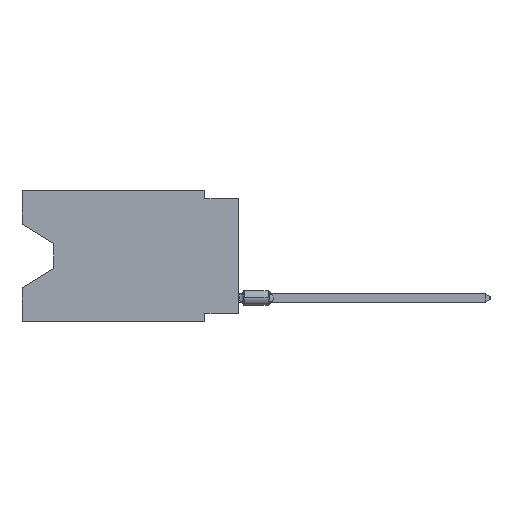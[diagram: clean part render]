
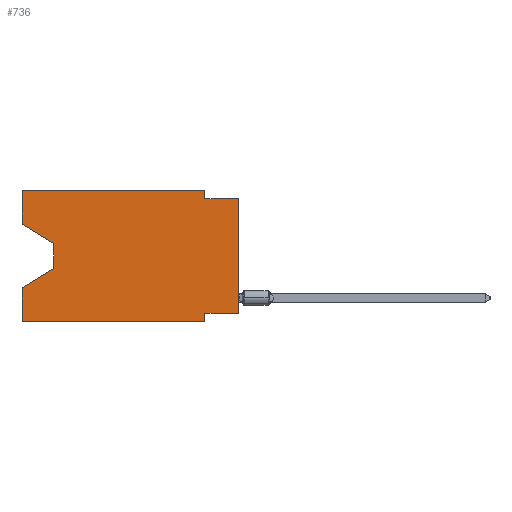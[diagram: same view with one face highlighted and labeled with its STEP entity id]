
A CAD part, left-side view. The second image highlights one B-rep face of the part: STEP entity #736.
In plain terms, the highlighted planar face has unit normal (-1, 0, 0).
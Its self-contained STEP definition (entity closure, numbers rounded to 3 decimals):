
#76 = CARTESIAN_POINT ( 'NONE',  ( 0., 13.97, -5.893 ) ) ;
#272 = VERTEX_POINT ( 'NONE', #35394 ) ;
#341 = CARTESIAN_POINT ( 'NONE',  ( 0., 0., -9.271 ) ) ;
#736 = ADVANCED_FACE ( 'NONE', ( #37414 ), #9203, .F. ) ;
#927 = CARTESIAN_POINT ( 'NONE',  ( 0., 16.383, 0. ) ) ;
#2332 = EDGE_CURVE ( 'NONE', #7585, #31117, #28357, .T. ) ;
#3087 = ORIENTED_EDGE ( 'NONE', *, *, #2332, .T. ) ;
#3330 = LINE ( 'NONE', #27055, #8369 ) ;
#6041 = CARTESIAN_POINT ( 'NONE',  ( 0., 16.383, -2.546 ) ) ;
#6537 = VERTEX_POINT ( 'NONE', #8122 ) ;
#6618 = LINE ( 'NONE', #6041, #17532 ) ;
#7310 = DIRECTION ( 'NONE',  ( 0., 0., -1. ) ) ;
#7585 = VERTEX_POINT ( 'NONE', #9325 ) ;
#7930 = EDGE_CURVE ( 'NONE', #23659, #9310, #6618, .T. ) ;
#7979 = ORIENTED_EDGE ( 'NONE', *, *, #18047, .F. ) ;
#8095 = AXIS2_PLACEMENT_3D ( 'NONE', #17760, #26076, #28738 ) ;
#8122 = CARTESIAN_POINT ( 'NONE',  ( 0., 2.54, -0.635 ) ) ;
#8369 = VECTOR ( 'NONE', #21730, 1000. ) ;
#8497 = DIRECTION ( 'NONE',  ( 0., 1., 0. ) ) ;
#8854 = DIRECTION ( 'NONE',  ( 0., -1., 0. ) ) ;
#9203 = PLANE ( 'NONE',  #8095 ) ;
#9310 = VERTEX_POINT ( 'NONE', #13341 ) ;
#9325 = CARTESIAN_POINT ( 'NONE',  ( 0., 13.97, -5.893 ) ) ;
#9574 = ORIENTED_EDGE ( 'NONE', *, *, #31504, .F. ) ;
#9662 = DIRECTION ( 'NONE',  ( 0., -0.855, -0.519 ) ) ;
#10177 = CARTESIAN_POINT ( 'NONE',  ( 0., 16.383, 0. ) ) ;
#10256 = CARTESIAN_POINT ( 'NONE',  ( 0., 13.97, -4.013 ) ) ;
#10736 = ORIENTED_EDGE ( 'NONE', *, *, #16623, .F. ) ;
#11288 = DIRECTION ( 'NONE',  ( 0., 0.855, -0.519 ) ) ;
#11717 = LINE ( 'NONE', #29138, #30243 ) ;
#13217 = EDGE_CURVE ( 'NONE', #18635, #31117, #26921, .T. ) ;
#13341 = CARTESIAN_POINT ( 'NONE',  ( 0., 13.97, -4.013 ) ) ;
#13473 = CARTESIAN_POINT ( 'NONE',  ( 0., 16.383, 0. ) ) ;
#13570 = EDGE_CURVE ( 'NONE', #24714, #31814, #32721, .T. ) ;
#13588 = VECTOR ( 'NONE', #15392, 1000. ) ;
#13828 = ORIENTED_EDGE ( 'NONE', *, *, #13217, .F. ) ;
#14167 = CARTESIAN_POINT ( 'NONE',  ( 0., 2.54, 0. ) ) ;
#14769 = CARTESIAN_POINT ( 'NONE',  ( 0., 16.383, -9.906 ) ) ;
#15392 = DIRECTION ( 'NONE',  ( 0., 0., 1. ) ) ;
#15533 = ORIENTED_EDGE ( 'NONE', *, *, #25763, .T. ) ;
#16104 = VECTOR ( 'NONE', #16131, 1000. ) ;
#16131 = DIRECTION ( 'NONE',  ( 0., 0., -1. ) ) ;
#16236 = DIRECTION ( 'NONE',  ( 0., 0., 1. ) ) ;
#16623 = EDGE_CURVE ( 'NONE', #34202, #24714, #34639, .T. ) ;
#17140 = ORIENTED_EDGE ( 'NONE', *, *, #31445, .T. ) ;
#17532 = VECTOR ( 'NONE', #9662, 1000. ) ;
#17760 = CARTESIAN_POINT ( 'NONE',  ( 0., 16.383, 0. ) ) ;
#18023 = VECTOR ( 'NONE', #34602, 1000. ) ;
#18047 = EDGE_CURVE ( 'NONE', #31237, #272, #27660, .T. ) ;
#18220 = EDGE_CURVE ( 'NONE', #34202, #36977, #33170, .T. ) ;
#18635 = VERTEX_POINT ( 'NONE', #14769 ) ;
#19332 = CARTESIAN_POINT ( 'NONE',  ( 0., 16.383, 0. ) ) ;
#19487 = ORIENTED_EDGE ( 'NONE', *, *, #27889, .F. ) ;
#19808 = CARTESIAN_POINT ( 'NONE',  ( 0., 16.383, -2.546 ) ) ;
#20255 = ORIENTED_EDGE ( 'NONE', *, *, #7930, .T. ) ;
#20990 = EDGE_CURVE ( 'NONE', #6537, #36977, #11717, .T. ) ;
#21642 = CARTESIAN_POINT ( 'NONE',  ( 0., 16.383, -7.36 ) ) ;
#21730 = DIRECTION ( 'NONE',  ( 0., -1., 0. ) ) ;
#21782 = DIRECTION ( 'NONE',  ( 0., 0., 1. ) ) ;
#22181 = VECTOR ( 'NONE', #11288, 1000. ) ;
#22882 = ORIENTED_EDGE ( 'NONE', *, *, #20990, .F. ) ;
#23065 = LINE ( 'NONE', #14167, #18023 ) ;
#23195 = VECTOR ( 'NONE', #24816, 1000. ) ;
#23658 = VECTOR ( 'NONE', #7310, 1000. ) ;
#23659 = VERTEX_POINT ( 'NONE', #19808 ) ;
#24136 = VECTOR ( 'NONE', #16236, 1000. ) ;
#24227 = CARTESIAN_POINT ( 'NONE',  ( 0., 2.54, -9.906 ) ) ;
#24304 = CARTESIAN_POINT ( 'NONE',  ( 0., 0., 0. ) ) ;
#24714 = VERTEX_POINT ( 'NONE', #30608 ) ;
#24816 = DIRECTION ( 'NONE',  ( 0., -1., 0. ) ) ;
#24842 = VECTOR ( 'NONE', #21782, 1000. ) ;
#25763 = EDGE_CURVE ( 'NONE', #9310, #7585, #36184, .T. ) ;
#26076 = DIRECTION ( 'NONE',  ( 1., 0., 0. ) ) ;
#26921 = LINE ( 'NONE', #927, #24842 ) ;
#27055 = CARTESIAN_POINT ( 'NONE',  ( 0., 16.383, -9.906 ) ) ;
#27435 = ORIENTED_EDGE ( 'NONE', *, *, #13570, .F. ) ;
#27660 = LINE ( 'NONE', #19332, #23195 ) ;
#27889 = EDGE_CURVE ( 'NONE', #272, #6537, #23065, .T. ) ;
#28357 = LINE ( 'NONE', #76, #22181 ) ;
#28738 = DIRECTION ( 'NONE',  ( 0., 0., -1. ) ) ;
#28955 = EDGE_LOOP ( 'NONE', ( #20255, #15533, #3087, #13828, #17140, #27435, #10736, #35342, #22882, #19487, #7979, #9574 ) ) ;
#29138 = CARTESIAN_POINT ( 'NONE',  ( 0., 0., -0.635 ) ) ;
#30012 = VECTOR ( 'NONE', #8497, 1000. ) ;
#30035 = CARTESIAN_POINT ( 'NONE',  ( 0., 0., -9.271 ) ) ;
#30243 = VECTOR ( 'NONE', #8854, 1000. ) ;
#30608 = CARTESIAN_POINT ( 'NONE',  ( 0., 2.54, -9.271 ) ) ;
#31117 = VERTEX_POINT ( 'NONE', #21642 ) ;
#31237 = VERTEX_POINT ( 'NONE', #13473 ) ;
#31445 = EDGE_CURVE ( 'NONE', #18635, #31814, #3330, .T. ) ;
#31504 = EDGE_CURVE ( 'NONE', #23659, #31237, #33455, .T. ) ;
#31814 = VERTEX_POINT ( 'NONE', #37385 ) ;
#31938 = CARTESIAN_POINT ( 'NONE',  ( 0., 0., -0.635 ) ) ;
#32721 = LINE ( 'NONE', #24227, #23658 ) ;
#33170 = LINE ( 'NONE', #24304, #13588 ) ;
#33455 = LINE ( 'NONE', #10177, #24136 ) ;
#34202 = VERTEX_POINT ( 'NONE', #30035 ) ;
#34602 = DIRECTION ( 'NONE',  ( 0., 0., -1. ) ) ;
#34639 = LINE ( 'NONE', #341, #30012 ) ;
#35342 = ORIENTED_EDGE ( 'NONE', *, *, #18220, .T. ) ;
#35394 = CARTESIAN_POINT ( 'NONE',  ( 0., 2.54, 0. ) ) ;
#36184 = LINE ( 'NONE', #10256, #16104 ) ;
#36977 = VERTEX_POINT ( 'NONE', #31938 ) ;
#37385 = CARTESIAN_POINT ( 'NONE',  ( 0., 2.54, -9.906 ) ) ;
#37414 = FACE_OUTER_BOUND ( 'NONE', #28955, .T. ) ;
